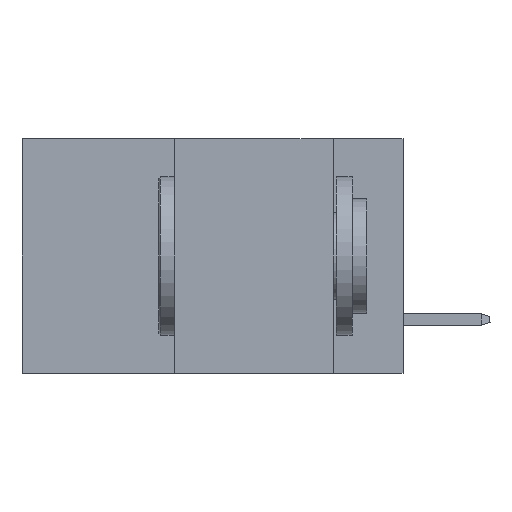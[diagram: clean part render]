
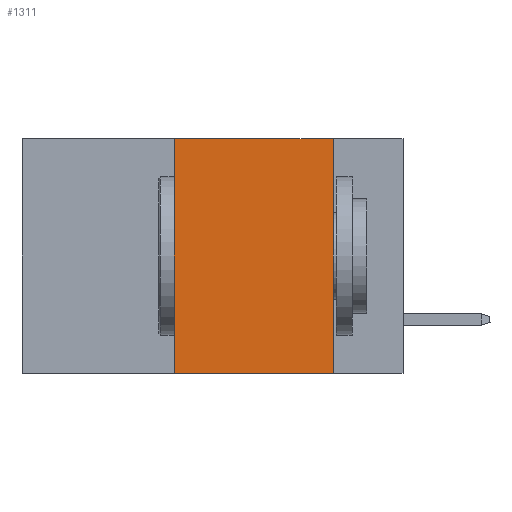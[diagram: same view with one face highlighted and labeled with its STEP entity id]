
A CAD part, left-side view. The second image highlights one B-rep face of the part: STEP entity #1311.
In plain terms, the highlighted planar face has unit normal (-1, 0, 0).
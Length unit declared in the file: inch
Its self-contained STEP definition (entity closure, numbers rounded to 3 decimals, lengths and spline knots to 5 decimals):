
#593 = CARTESIAN_POINT ( 'NONE',  ( 0., 0.36, 0. ) ) ;
#620 = EDGE_CURVE ( 'NONE', #12877, #20656, #5940, .T. ) ;
#1310 = EDGE_CURVE ( 'NONE', #12877, #4456, #14383, .T. ) ;
#1311 = ADVANCED_FACE ( 'NONE', ( #13463 ), #10008, .F. ) ;
#1380 = EDGE_CURVE ( 'NONE', #13180, #20656, #5786, .T. ) ;
#2735 = CARTESIAN_POINT ( 'NONE',  ( 0., 0.11, 0. ) ) ;
#3546 = DIRECTION ( 'NONE',  ( 0., -1., 0. ) ) ;
#3553 = ORIENTED_EDGE ( 'NONE', *, *, #620, .T. ) ;
#3833 = CARTESIAN_POINT ( 'NONE',  ( 0., 0.36, -0.37 ) ) ;
#4124 = CARTESIAN_POINT ( 'NONE',  ( 0., 0.11, 0. ) ) ;
#4456 = VERTEX_POINT ( 'NONE', #15646 ) ;
#4810 = DIRECTION ( 'NONE',  ( 1., 0., 0. ) ) ;
#4920 = DIRECTION ( 'NONE',  ( 0., 0., -1. ) ) ;
#5028 = CARTESIAN_POINT ( 'NONE',  ( 0., 0.6, 0. ) ) ;
#5786 = LINE ( 'NONE', #4124, #12821 ) ;
#5940 = LINE ( 'NONE', #17785, #20189 ) ;
#7630 = CARTESIAN_POINT ( 'NONE',  ( 0., 0.11, -0.37 ) ) ;
#9345 = ORIENTED_EDGE ( 'NONE', *, *, #9835, .F. ) ;
#9835 = EDGE_CURVE ( 'NONE', #4456, #13180, #13888, .T. ) ;
#9974 = AXIS2_PLACEMENT_3D ( 'NONE', #5028, #4810, #4920 ) ;
#10008 = PLANE ( 'NONE',  #9974 ) ;
#10975 = EDGE_LOOP ( 'NONE', ( #18773, #9345, #19541, #3553 ) ) ;
#12393 = DIRECTION ( 'NONE',  ( 0., -1., 0. ) ) ;
#12821 = VECTOR ( 'NONE', #14333, 39.37008 ) ;
#12877 = VERTEX_POINT ( 'NONE', #3833 ) ;
#13180 = VERTEX_POINT ( 'NONE', #2735 ) ;
#13463 = FACE_OUTER_BOUND ( 'NONE', #10975, .T. ) ;
#13669 = CARTESIAN_POINT ( 'NONE',  ( 0., 0.6, 0. ) ) ;
#13888 = LINE ( 'NONE', #13669, #18910 ) ;
#14333 = DIRECTION ( 'NONE',  ( 0., 0., -1. ) ) ;
#14383 = LINE ( 'NONE', #593, #20941 ) ;
#15646 = CARTESIAN_POINT ( 'NONE',  ( 0., 0.36, 0. ) ) ;
#17785 = CARTESIAN_POINT ( 'NONE',  ( 0., 0.6, -0.37 ) ) ;
#18773 = ORIENTED_EDGE ( 'NONE', *, *, #1380, .F. ) ;
#18910 = VECTOR ( 'NONE', #3546, 39.37008 ) ;
#19541 = ORIENTED_EDGE ( 'NONE', *, *, #1310, .F. ) ;
#19575 = DIRECTION ( 'NONE',  ( 0., 0., 1. ) ) ;
#20189 = VECTOR ( 'NONE', #12393, 39.37008 ) ;
#20656 = VERTEX_POINT ( 'NONE', #7630 ) ;
#20941 = VECTOR ( 'NONE', #19575, 39.37008 ) ;
